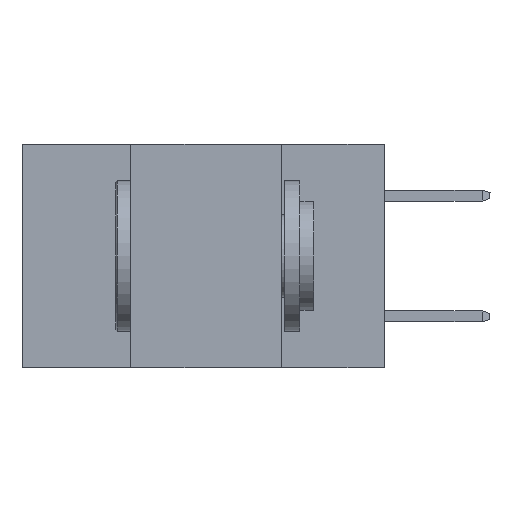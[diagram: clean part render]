
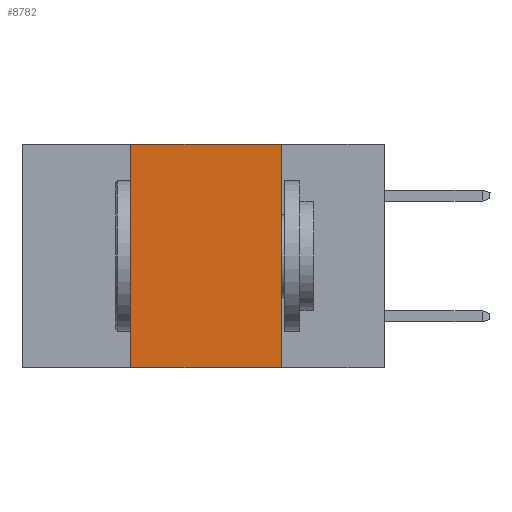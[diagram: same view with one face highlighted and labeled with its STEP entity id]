
A CAD part, left-side view. The second image highlights one B-rep face of the part: STEP entity #8782.
In plain terms, the highlighted planar face has unit normal (-1, 0, 0).
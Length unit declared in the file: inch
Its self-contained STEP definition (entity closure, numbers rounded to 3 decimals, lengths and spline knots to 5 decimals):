
#327 = ORIENTED_EDGE ( 'NONE', *, *, #24230, .F. ) ;
#1760 = DIRECTION ( 'NONE',  ( 0., -1., 0. ) ) ;
#1923 = ORIENTED_EDGE ( 'NONE', *, *, #20677, .F. ) ;
#4072 = LINE ( 'NONE', #8100, #16050 ) ;
#4094 = DIRECTION ( 'NONE',  ( 0., 0., 1. ) ) ;
#4862 = PLANE ( 'NONE',  #23171 ) ;
#6332 = VERTEX_POINT ( 'NONE', #19537 ) ;
#6351 = VECTOR ( 'NONE', #1760, 39.37008 ) ;
#6985 = CARTESIAN_POINT ( 'NONE',  ( 0., 0.6, 0. ) ) ;
#7023 = LINE ( 'NONE', #24517, #6351 ) ;
#8100 = CARTESIAN_POINT ( 'NONE',  ( 0., 0.6, -0.37 ) ) ;
#8195 = FACE_OUTER_BOUND ( 'NONE', #15451, .T. ) ;
#8782 = ADVANCED_FACE ( 'NONE', ( #8195 ), #4862, .F. ) ;
#9582 = DIRECTION ( 'NONE',  ( 1., 0., 0. ) ) ;
#12223 = CARTESIAN_POINT ( 'NONE',  ( 0., 0.17, 0. ) ) ;
#12558 = CARTESIAN_POINT ( 'NONE',  ( 0., 0.42, -0.37 ) ) ;
#13373 = CARTESIAN_POINT ( 'NONE',  ( 0., 0.17, -0.37 ) ) ;
#13460 = VERTEX_POINT ( 'NONE', #16333 ) ;
#14730 = VERTEX_POINT ( 'NONE', #12558 ) ;
#15451 = EDGE_LOOP ( 'NONE', ( #1923, #17517, #327, #24990 ) ) ;
#16050 = VECTOR ( 'NONE', #21431, 39.37008 ) ;
#16333 = CARTESIAN_POINT ( 'NONE',  ( 0., 0.17, 0. ) ) ;
#17517 = ORIENTED_EDGE ( 'NONE', *, *, #22873, .F. ) ;
#17761 = VERTEX_POINT ( 'NONE', #13373 ) ;
#18054 = VECTOR ( 'NONE', #23355, 39.37008 ) ;
#18867 = VECTOR ( 'NONE', #4094, 39.37008 ) ;
#19483 = CARTESIAN_POINT ( 'NONE',  ( 0., 0.42, 0. ) ) ;
#19537 = CARTESIAN_POINT ( 'NONE',  ( 0., 0.42, 0. ) ) ;
#19539 = EDGE_CURVE ( 'NONE', #14730, #17761, #4072, .T. ) ;
#20231 = DIRECTION ( 'NONE',  ( 0., 0., -1. ) ) ;
#20456 = LINE ( 'NONE', #12223, #18054 ) ;
#20677 = EDGE_CURVE ( 'NONE', #13460, #17761, #20456, .T. ) ;
#21431 = DIRECTION ( 'NONE',  ( 0., -1., 0. ) ) ;
#22873 = EDGE_CURVE ( 'NONE', #6332, #13460, #7023, .T. ) ;
#23171 = AXIS2_PLACEMENT_3D ( 'NONE', #6985, #9582, #20231 ) ;
#23355 = DIRECTION ( 'NONE',  ( 0., 0., -1. ) ) ;
#24230 = EDGE_CURVE ( 'NONE', #14730, #6332, #24658, .T. ) ;
#24517 = CARTESIAN_POINT ( 'NONE',  ( 0., 0.6, 0. ) ) ;
#24658 = LINE ( 'NONE', #19483, #18867 ) ;
#24990 = ORIENTED_EDGE ( 'NONE', *, *, #19539, .T. ) ;
